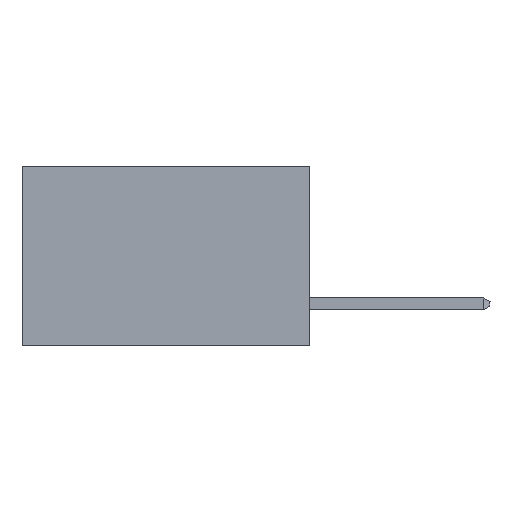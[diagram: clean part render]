
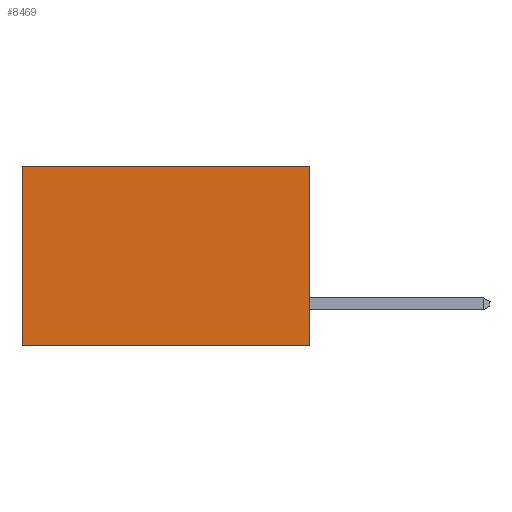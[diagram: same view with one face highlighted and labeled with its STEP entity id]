
A CAD part, left-side view. The second image highlights one B-rep face of the part: STEP entity #8469.
In plain terms, the highlighted planar face has unit normal (-1, 0, 0).
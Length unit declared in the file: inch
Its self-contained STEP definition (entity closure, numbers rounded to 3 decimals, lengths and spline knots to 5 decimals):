
#1346 = VECTOR ( 'NONE', #8988, 39.37008 ) ;
#1868 = LINE ( 'NONE', #5428, #14390 ) ;
#1889 = ORIENTED_EDGE ( 'NONE', *, *, #11550, .T. ) ;
#2597 = LINE ( 'NONE', #5486, #1346 ) ;
#2906 = EDGE_CURVE ( 'NONE', #6590, #5154, #9461, .T. ) ;
#2992 = VERTEX_POINT ( 'NONE', #10729 ) ;
#3446 = PLANE ( 'NONE',  #13103 ) ;
#3731 = EDGE_LOOP ( 'NONE', ( #5469, #9742, #11458, #1889 ) ) ;
#3779 = DIRECTION ( 'NONE',  ( 0., 0., -1. ) ) ;
#4263 = EDGE_CURVE ( 'NONE', #14232, #2992, #2597, .T. ) ;
#4603 = CARTESIAN_POINT ( 'NONE',  ( 0.2875, 0., -0.375 ) ) ;
#5154 = VERTEX_POINT ( 'NONE', #7851 ) ;
#5428 = CARTESIAN_POINT ( 'NONE',  ( 0.2875, 0., 0. ) ) ;
#5469 = ORIENTED_EDGE ( 'NONE', *, *, #4263, .T. ) ;
#5486 = CARTESIAN_POINT ( 'NONE',  ( 0.2875, 0.6, -0.375 ) ) ;
#5569 = DIRECTION ( 'NONE',  ( 1., 0., 0. ) ) ;
#5860 = CARTESIAN_POINT ( 'NONE',  ( 0.2875, 0.6, 0. ) ) ;
#6590 = VERTEX_POINT ( 'NONE', #10703 ) ;
#6668 = FACE_OUTER_BOUND ( 'NONE', #3731, .T. ) ;
#6767 = DIRECTION ( 'NONE',  ( 0., 0., -1. ) ) ;
#7851 = CARTESIAN_POINT ( 'NONE',  ( 0.2875, 0., -0.375 ) ) ;
#8288 = CARTESIAN_POINT ( 'NONE',  ( 0.2875, 0., -0.375 ) ) ;
#8469 = ADVANCED_FACE ( 'NONE', ( #6668 ), #3446, .F. ) ;
#8659 = CARTESIAN_POINT ( 'NONE',  ( 0.2875, 0., -0.375 ) ) ;
#8988 = DIRECTION ( 'NONE',  ( 0., 0., -1. ) ) ;
#9261 = VECTOR ( 'NONE', #9902, 39.37008 ) ;
#9461 = LINE ( 'NONE', #8288, #14081 ) ;
#9742 = ORIENTED_EDGE ( 'NONE', *, *, #13849, .F. ) ;
#9902 = DIRECTION ( 'NONE',  ( 0., 1., 0. ) ) ;
#10694 = LINE ( 'NONE', #8659, #9261 ) ;
#10703 = CARTESIAN_POINT ( 'NONE',  ( 0.2875, 0., 0. ) ) ;
#10729 = CARTESIAN_POINT ( 'NONE',  ( 0.2875, 0.6, -0.375 ) ) ;
#11458 = ORIENTED_EDGE ( 'NONE', *, *, #2906, .F. ) ;
#11550 = EDGE_CURVE ( 'NONE', #6590, #14232, #1868, .T. ) ;
#12341 = DIRECTION ( 'NONE',  ( 0., 1., 0. ) ) ;
#13103 = AXIS2_PLACEMENT_3D ( 'NONE', #4603, #5569, #6767 ) ;
#13849 = EDGE_CURVE ( 'NONE', #5154, #2992, #10694, .T. ) ;
#14081 = VECTOR ( 'NONE', #3779, 39.37008 ) ;
#14232 = VERTEX_POINT ( 'NONE', #5860 ) ;
#14390 = VECTOR ( 'NONE', #12341, 39.37008 ) ;
